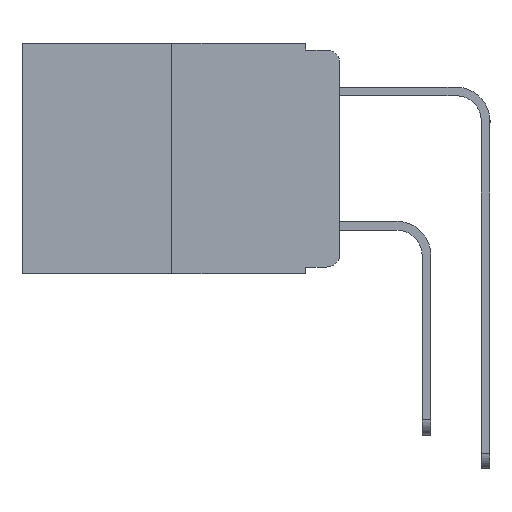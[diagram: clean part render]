
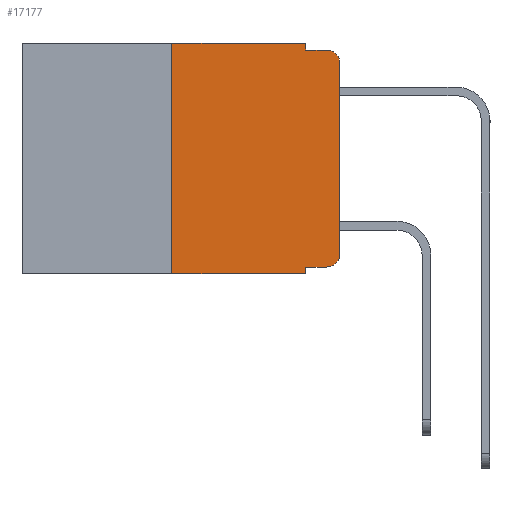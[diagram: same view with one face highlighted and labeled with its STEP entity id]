
A CAD part, left-side view. The second image highlights one B-rep face of the part: STEP entity #17177.
In plain terms, the highlighted planar face has unit normal (-1, 0, 0).
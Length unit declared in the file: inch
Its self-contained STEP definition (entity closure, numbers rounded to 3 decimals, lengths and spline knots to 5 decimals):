
#431 = VERTEX_POINT ( 'NONE', #11484 ) ;
#471 = VERTEX_POINT ( 'NONE', #1890 ) ;
#815 = VECTOR ( 'NONE', #12065, 39.37008 ) ;
#940 = DIRECTION ( 'NONE',  ( 0., 0., -1. ) ) ;
#1669 = EDGE_CURVE ( 'NONE', #12921, #13996, #16859, .T. ) ;
#1890 = CARTESIAN_POINT ( 'NONE',  ( 0., 0.051, -0.343 ) ) ;
#2041 = CARTESIAN_POINT ( 'NONE',  ( 0., 0.02, -0.313 ) ) ;
#2469 = CARTESIAN_POINT ( 'NONE',  ( 0., 0.051, 0. ) ) ;
#2611 = LINE ( 'NONE', #12340, #10960 ) ;
#3270 = CARTESIAN_POINT ( 'NONE',  ( 0., 0.051, -0.01 ) ) ;
#3403 = DIRECTION ( 'NONE',  ( -1., 0., 0. ) ) ;
#3599 = CARTESIAN_POINT ( 'NONE',  ( 0., 0.051, 0. ) ) ;
#3790 = VERTEX_POINT ( 'NONE', #18719 ) ;
#3935 = EDGE_CURVE ( 'NONE', #3790, #12921, #6524, .T. ) ;
#4230 = CARTESIAN_POINT ( 'NONE',  ( 0., 0.02, -0.333 ) ) ;
#4574 = LINE ( 'NONE', #2469, #20503 ) ;
#4973 = CARTESIAN_POINT ( 'NONE',  ( 0., 0.25, 0. ) ) ;
#5248 = ORIENTED_EDGE ( 'NONE', *, *, #18219, .T. ) ;
#5374 = DIRECTION ( 'NONE',  ( 0., -1., 0. ) ) ;
#5611 = VERTEX_POINT ( 'NONE', #16875 ) ;
#6006 = FACE_OUTER_BOUND ( 'NONE', #9542, .T. ) ;
#6132 = EDGE_CURVE ( 'NONE', #3790, #471, #20308, .T. ) ;
#6171 = VERTEX_POINT ( 'NONE', #19668 ) ;
#6524 = LINE ( 'NONE', #8851, #10957 ) ;
#7265 = EDGE_CURVE ( 'NONE', #5611, #431, #12854, .T. ) ;
#7623 = ORIENTED_EDGE ( 'NONE', *, *, #13867, .T. ) ;
#8343 = VECTOR ( 'NONE', #15050, 39.37008 ) ;
#8457 = DIRECTION ( 'NONE',  ( 0., 0., 1. ) ) ;
#8811 = DIRECTION ( 'NONE',  ( 0., 0., -1. ) ) ;
#8851 = CARTESIAN_POINT ( 'NONE',  ( 0., 0.051, -0.333 ) ) ;
#9497 = VERTEX_POINT ( 'NONE', #12728 ) ;
#9542 = EDGE_LOOP ( 'NONE', ( #19709, #7623, #20168, #16671, #13010, #13537, #5248, #18088, #14991, #11254 ) ) ;
#10633 = EDGE_CURVE ( 'NONE', #6171, #11949, #4574, .T. ) ;
#10957 = VECTOR ( 'NONE', #5374, 39.37008 ) ;
#10960 = VECTOR ( 'NONE', #18488, 39.37008 ) ;
#10977 = DIRECTION ( 'NONE',  ( 1., 0., 0. ) ) ;
#10999 = CIRCLE ( 'NONE', #12266, 0.02 ) ;
#11037 = LINE ( 'NONE', #12553, #19270 ) ;
#11254 = ORIENTED_EDGE ( 'NONE', *, *, #1669, .T. ) ;
#11425 = AXIS2_PLACEMENT_3D ( 'NONE', #2041, #18217, #8811 ) ;
#11484 = CARTESIAN_POINT ( 'NONE',  ( 0., 0.25, 0. ) ) ;
#11723 = VECTOR ( 'NONE', #8457, 39.37008 ) ;
#11949 = VERTEX_POINT ( 'NONE', #3270 ) ;
#12065 = DIRECTION ( 'NONE',  ( 0., -1., 0. ) ) ;
#12266 = AXIS2_PLACEMENT_3D ( 'NONE', #13293, #3403, #14866 ) ;
#12340 = CARTESIAN_POINT ( 'NONE',  ( 0., 0.473, -0.343 ) ) ;
#12553 = CARTESIAN_POINT ( 'NONE',  ( 0., 0.473, 0. ) ) ;
#12728 = CARTESIAN_POINT ( 'NONE',  ( 0., 0.02, -0.01 ) ) ;
#12782 = EDGE_CURVE ( 'NONE', #11949, #9497, #18582, .T. ) ;
#12854 = LINE ( 'NONE', #4973, #20023 ) ;
#12921 = VERTEX_POINT ( 'NONE', #4230 ) ;
#12937 = EDGE_CURVE ( 'NONE', #431, #6171, #11037, .T. ) ;
#13010 = ORIENTED_EDGE ( 'NONE', *, *, #12937, .F. ) ;
#13293 = CARTESIAN_POINT ( 'NONE',  ( 0., 0.02, -0.03 ) ) ;
#13299 = DIRECTION ( 'NONE',  ( 0., 0., 1. ) ) ;
#13537 = ORIENTED_EDGE ( 'NONE', *, *, #7265, .F. ) ;
#13867 = EDGE_CURVE ( 'NONE', #19653, #9497, #10999, .T. ) ;
#13947 = DIRECTION ( 'NONE',  ( 0., 0., -1. ) ) ;
#13996 = VERTEX_POINT ( 'NONE', #19635 ) ;
#14266 = CARTESIAN_POINT ( 'NONE',  ( 0., 0., -0.03 ) ) ;
#14848 = CARTESIAN_POINT ( 'NONE',  ( 0., 0., 0. ) ) ;
#14866 = DIRECTION ( 'NONE',  ( 0., 0., -1. ) ) ;
#14991 = ORIENTED_EDGE ( 'NONE', *, *, #3935, .T. ) ;
#15050 = DIRECTION ( 'NONE',  ( 0., 0., -1. ) ) ;
#15250 = CARTESIAN_POINT ( 'NONE',  ( 0., 0.051, -0.01 ) ) ;
#15675 = CARTESIAN_POINT ( 'NONE',  ( 0., 0.473, 0. ) ) ;
#15923 = LINE ( 'NONE', #14848, #11723 ) ;
#16671 = ORIENTED_EDGE ( 'NONE', *, *, #10633, .F. ) ;
#16859 = CIRCLE ( 'NONE', #11425, 0.02 ) ;
#16875 = CARTESIAN_POINT ( 'NONE',  ( 0., 0.25, -0.343 ) ) ;
#17177 = ADVANCED_FACE ( 'NONE', ( #6006 ), #20215, .F. ) ;
#17969 = EDGE_CURVE ( 'NONE', #13996, #19653, #15923, .T. ) ;
#18088 = ORIENTED_EDGE ( 'NONE', *, *, #6132, .F. ) ;
#18217 = DIRECTION ( 'NONE',  ( -1., 0., 0. ) ) ;
#18219 = EDGE_CURVE ( 'NONE', #5611, #471, #2611, .T. ) ;
#18488 = DIRECTION ( 'NONE',  ( 0., -1., 0. ) ) ;
#18582 = LINE ( 'NONE', #15250, #815 ) ;
#18681 = DIRECTION ( 'NONE',  ( 0., -1., 0. ) ) ;
#18719 = CARTESIAN_POINT ( 'NONE',  ( 0., 0.051, -0.333 ) ) ;
#19028 = AXIS2_PLACEMENT_3D ( 'NONE', #15675, #10977, #940 ) ;
#19270 = VECTOR ( 'NONE', #18681, 39.37008 ) ;
#19635 = CARTESIAN_POINT ( 'NONE',  ( 0., 0., -0.313 ) ) ;
#19653 = VERTEX_POINT ( 'NONE', #14266 ) ;
#19668 = CARTESIAN_POINT ( 'NONE',  ( 0., 0.051, 0. ) ) ;
#19709 = ORIENTED_EDGE ( 'NONE', *, *, #17969, .T. ) ;
#20023 = VECTOR ( 'NONE', #13299, 39.37008 ) ;
#20168 = ORIENTED_EDGE ( 'NONE', *, *, #12782, .F. ) ;
#20215 = PLANE ( 'NONE',  #19028 ) ;
#20308 = LINE ( 'NONE', #3599, #8343 ) ;
#20503 = VECTOR ( 'NONE', #13947, 39.37008 ) ;
